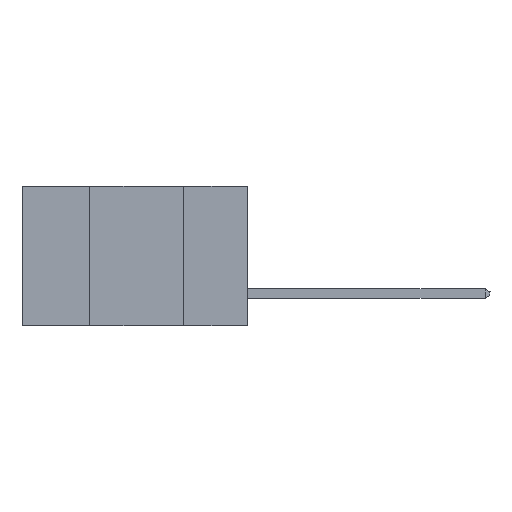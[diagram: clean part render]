
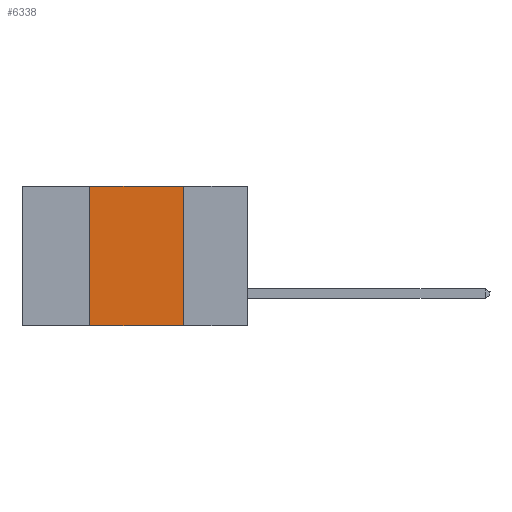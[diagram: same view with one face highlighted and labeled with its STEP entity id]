
A CAD part, left-side view. The second image highlights one B-rep face of the part: STEP entity #6338.
In plain terms, the highlighted planar face has unit normal (-1, 0, 0).
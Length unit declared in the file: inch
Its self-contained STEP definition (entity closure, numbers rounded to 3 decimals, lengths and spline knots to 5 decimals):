
#606 = FACE_OUTER_BOUND ( 'NONE', #12552, .T. ) ;
#2558 = DIRECTION ( 'NONE',  ( 0., -1., 0. ) ) ;
#2683 = ORIENTED_EDGE ( 'NONE', *, *, #10107, .F. ) ;
#2870 = CARTESIAN_POINT ( 'NONE',  ( 0., 0.17, -0.37 ) ) ;
#3052 = AXIS2_PLACEMENT_3D ( 'NONE', #4508, #13363, #8296 ) ;
#4080 = EDGE_CURVE ( 'NONE', #23003, #15382, #8439, .T. ) ;
#4197 = CARTESIAN_POINT ( 'NONE',  ( 0., 0.17, 0. ) ) ;
#4508 = CARTESIAN_POINT ( 'NONE',  ( 0., 0.6, 0. ) ) ;
#5781 = VERTEX_POINT ( 'NONE', #17836 ) ;
#5934 = EDGE_CURVE ( 'NONE', #13765, #23003, #20331, .T. ) ;
#6338 = ADVANCED_FACE ( 'NONE', ( #606 ), #20732, .F. ) ;
#6760 = LINE ( 'NONE', #13865, #20927 ) ;
#8296 = DIRECTION ( 'NONE',  ( 0., 0., -1. ) ) ;
#8439 = LINE ( 'NONE', #2870, #11391 ) ;
#8793 = ORIENTED_EDGE ( 'NONE', *, *, #15020, .T. ) ;
#10079 = DIRECTION ( 'NONE',  ( 0., 0., -1. ) ) ;
#10107 = EDGE_CURVE ( 'NONE', #5781, #13765, #11790, .T. ) ;
#10673 = ORIENTED_EDGE ( 'NONE', *, *, #4080, .F. ) ;
#10729 = VECTOR ( 'NONE', #13437, 39.37008 ) ;
#11391 = VECTOR ( 'NONE', #10079, 39.37008 ) ;
#11544 = CARTESIAN_POINT ( 'NONE',  ( 0., 0.42, -0.37 ) ) ;
#11570 = CARTESIAN_POINT ( 'NONE',  ( 0., 0.17, -0.37 ) ) ;
#11790 = LINE ( 'NONE', #11544, #10729 ) ;
#12552 = EDGE_LOOP ( 'NONE', ( #10673, #18016, #2683, #8793 ) ) ;
#13363 = DIRECTION ( 'NONE',  ( 1., 0., 0. ) ) ;
#13426 = VECTOR ( 'NONE', #2558, 39.37008 ) ;
#13437 = DIRECTION ( 'NONE',  ( 0., 0., 1. ) ) ;
#13765 = VERTEX_POINT ( 'NONE', #15183 ) ;
#13865 = CARTESIAN_POINT ( 'NONE',  ( 0., 0.6, -0.37 ) ) ;
#15020 = EDGE_CURVE ( 'NONE', #5781, #15382, #6760, .T. ) ;
#15183 = CARTESIAN_POINT ( 'NONE',  ( 0., 0.42, 0. ) ) ;
#15382 = VERTEX_POINT ( 'NONE', #11570 ) ;
#17836 = CARTESIAN_POINT ( 'NONE',  ( 0., 0.42, -0.37 ) ) ;
#18016 = ORIENTED_EDGE ( 'NONE', *, *, #5934, .F. ) ;
#18546 = CARTESIAN_POINT ( 'NONE',  ( 0., 0.6, 0. ) ) ;
#20331 = LINE ( 'NONE', #18546, #13426 ) ;
#20732 = PLANE ( 'NONE',  #3052 ) ;
#20927 = VECTOR ( 'NONE', #21094, 39.37008 ) ;
#21094 = DIRECTION ( 'NONE',  ( 0., -1., 0. ) ) ;
#23003 = VERTEX_POINT ( 'NONE', #4197 ) ;
